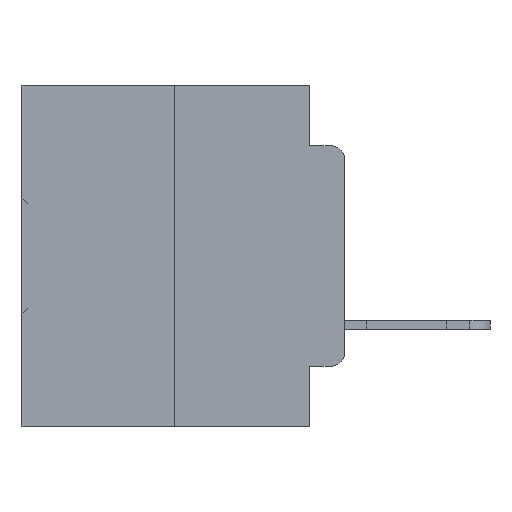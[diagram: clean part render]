
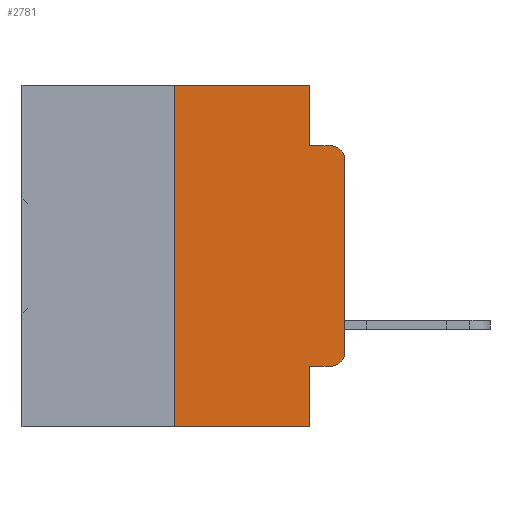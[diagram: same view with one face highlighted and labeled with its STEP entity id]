
A CAD part, left-side view. The second image highlights one B-rep face of the part: STEP entity #2781.
In plain terms, the highlighted planar face has unit normal (-1, 0, 0).
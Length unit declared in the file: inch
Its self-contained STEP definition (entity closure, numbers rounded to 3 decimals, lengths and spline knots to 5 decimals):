
#951 = EDGE_LOOP ( 'NONE', ( #16702, #34845, #14165, #1752, #12583, #24520, #26987, #28486, #2796, #16940 ) ) ;
#1752 = ORIENTED_EDGE ( 'NONE', *, *, #7060, .F. ) ;
#1997 = DIRECTION ( 'NONE',  ( -1., 0., 0. ) ) ;
#2239 = LINE ( 'NONE', #32340, #24091 ) ;
#2675 = DIRECTION ( 'NONE',  ( 0., 0., 1. ) ) ;
#2781 = ADVANCED_FACE ( 'NONE', ( #27780 ), #6393, .F. ) ;
#2796 = ORIENTED_EDGE ( 'NONE', *, *, #31433, .T. ) ;
#2851 = CARTESIAN_POINT ( 'NONE',  ( 0., 0., 0. ) ) ;
#3292 = VERTEX_POINT ( 'NONE', #24514 ) ;
#4327 = LINE ( 'NONE', #14960, #11326 ) ;
#4778 = LINE ( 'NONE', #31733, #27092 ) ;
#4791 = CARTESIAN_POINT ( 'NONE',  ( 0., 0.25, -0.5 ) ) ;
#5276 = VERTEX_POINT ( 'NONE', #4791 ) ;
#6227 = DIRECTION ( 'NONE',  ( 0., 0., -1. ) ) ;
#6255 = VECTOR ( 'NONE', #18401, 39.37008 ) ;
#6272 = DIRECTION ( 'NONE',  ( 1., 0., 0. ) ) ;
#6393 = PLANE ( 'NONE',  #18768 ) ;
#6863 = CARTESIAN_POINT ( 'NONE',  ( 0., 0., -0.3915 ) ) ;
#7060 = EDGE_CURVE ( 'NONE', #3292, #7472, #4778, .T. ) ;
#7232 = CARTESIAN_POINT ( 'NONE',  ( 0., 0.473, 0. ) ) ;
#7472 = VERTEX_POINT ( 'NONE', #17332 ) ;
#7509 = VERTEX_POINT ( 'NONE', #14295 ) ;
#8994 = LINE ( 'NONE', #24898, #15753 ) ;
#8995 = CARTESIAN_POINT ( 'NONE',  ( 0., 0.02, -0.4115 ) ) ;
#10977 = EDGE_CURVE ( 'NONE', #7472, #30550, #12567, .T. ) ;
#11326 = VECTOR ( 'NONE', #28295, 39.37008 ) ;
#12567 = LINE ( 'NONE', #21452, #18228 ) ;
#12583 = ORIENTED_EDGE ( 'NONE', *, *, #30426, .F. ) ;
#12823 = VERTEX_POINT ( 'NONE', #28527 ) ;
#12955 = EDGE_CURVE ( 'NONE', #27573, #30550, #14167, .T. ) ;
#13745 = CARTESIAN_POINT ( 'NONE',  ( 0., 0., -0.1085 ) ) ;
#13796 = VERTEX_POINT ( 'NONE', #8995 ) ;
#14165 = ORIENTED_EDGE ( 'NONE', *, *, #10977, .F. ) ;
#14167 = CIRCLE ( 'NONE', #18147, 0.02 ) ;
#14295 = CARTESIAN_POINT ( 'NONE',  ( 0., 0.051, -0.4115 ) ) ;
#14604 = EDGE_CURVE ( 'NONE', #5276, #29363, #8994, .T. ) ;
#14680 = VECTOR ( 'NONE', #32801, 39.37008 ) ;
#14824 = EDGE_CURVE ( 'NONE', #32777, #27573, #23410, .T. ) ;
#14960 = CARTESIAN_POINT ( 'NONE',  ( 0., 0.473, 0. ) ) ;
#15619 = CARTESIAN_POINT ( 'NONE',  ( 0., 0.051, -0.4115 ) ) ;
#15753 = VECTOR ( 'NONE', #24825, 39.37008 ) ;
#16702 = ORIENTED_EDGE ( 'NONE', *, *, #14824, .T. ) ;
#16940 = ORIENTED_EDGE ( 'NONE', *, *, #22790, .T. ) ;
#17071 = VECTOR ( 'NONE', #2675, 39.37008 ) ;
#17332 = CARTESIAN_POINT ( 'NONE',  ( 0., 0.051, -0.0885 ) ) ;
#18147 = AXIS2_PLACEMENT_3D ( 'NONE', #25422, #25384, #25356 ) ;
#18228 = VECTOR ( 'NONE', #21155, 39.37008 ) ;
#18401 = DIRECTION ( 'NONE',  ( 0., -1., 0. ) ) ;
#18768 = AXIS2_PLACEMENT_3D ( 'NONE', #7232, #6272, #6227 ) ;
#19356 = CARTESIAN_POINT ( 'NONE',  ( 0., 0.02, -0.3915 ) ) ;
#19357 = DIRECTION ( 'NONE',  ( 0., 0., -1. ) ) ;
#20350 = LINE ( 'NONE', #15619, #6255 ) ;
#20753 = CARTESIAN_POINT ( 'NONE',  ( 0., 0.02, -0.0885 ) ) ;
#21155 = DIRECTION ( 'NONE',  ( 0., -1., 0. ) ) ;
#21452 = CARTESIAN_POINT ( 'NONE',  ( 0., 0.051, -0.0885 ) ) ;
#22070 = DIRECTION ( 'NONE',  ( 0., 0., -1. ) ) ;
#22790 = EDGE_CURVE ( 'NONE', #13796, #32777, #27813, .T. ) ;
#23410 = LINE ( 'NONE', #2851, #17071 ) ;
#24091 = VECTOR ( 'NONE', #19357, 39.37008 ) ;
#24514 = CARTESIAN_POINT ( 'NONE',  ( 0., 0.051, 0. ) ) ;
#24520 = ORIENTED_EDGE ( 'NONE', *, *, #34691, .F. ) ;
#24825 = DIRECTION ( 'NONE',  ( 0., -1., 0. ) ) ;
#24898 = CARTESIAN_POINT ( 'NONE',  ( 0., 0.473, -0.5 ) ) ;
#25356 = DIRECTION ( 'NONE',  ( 0., 0., -1. ) ) ;
#25384 = DIRECTION ( 'NONE',  ( -1., 0., 0. ) ) ;
#25422 = CARTESIAN_POINT ( 'NONE',  ( 0., 0.02, -0.1085 ) ) ;
#26987 = ORIENTED_EDGE ( 'NONE', *, *, #14604, .T. ) ;
#27092 = VECTOR ( 'NONE', #31446, 39.37008 ) ;
#27573 = VERTEX_POINT ( 'NONE', #13745 ) ;
#27780 = FACE_OUTER_BOUND ( 'NONE', #951, .T. ) ;
#27813 = CIRCLE ( 'NONE', #31502, 0.02 ) ;
#28295 = DIRECTION ( 'NONE',  ( 0., -1., 0. ) ) ;
#28486 = ORIENTED_EDGE ( 'NONE', *, *, #33092, .F. ) ;
#28527 = CARTESIAN_POINT ( 'NONE',  ( 0., 0.25, 0. ) ) ;
#29363 = VERTEX_POINT ( 'NONE', #29699 ) ;
#29699 = CARTESIAN_POINT ( 'NONE',  ( 0., 0.051, -0.5 ) ) ;
#30426 = EDGE_CURVE ( 'NONE', #12823, #3292, #4327, .T. ) ;
#30481 = LINE ( 'NONE', #35126, #14680 ) ;
#30550 = VERTEX_POINT ( 'NONE', #20753 ) ;
#31433 = EDGE_CURVE ( 'NONE', #7509, #13796, #20350, .T. ) ;
#31446 = DIRECTION ( 'NONE',  ( 0., 0., -1. ) ) ;
#31502 = AXIS2_PLACEMENT_3D ( 'NONE', #19356, #1997, #22070 ) ;
#31733 = CARTESIAN_POINT ( 'NONE',  ( 0., 0.051, 0. ) ) ;
#32340 = CARTESIAN_POINT ( 'NONE',  ( 0., 0.051, 0. ) ) ;
#32777 = VERTEX_POINT ( 'NONE', #6863 ) ;
#32801 = DIRECTION ( 'NONE',  ( 0., 0., 1. ) ) ;
#33092 = EDGE_CURVE ( 'NONE', #7509, #29363, #2239, .T. ) ;
#34691 = EDGE_CURVE ( 'NONE', #5276, #12823, #30481, .T. ) ;
#34845 = ORIENTED_EDGE ( 'NONE', *, *, #12955, .T. ) ;
#35126 = CARTESIAN_POINT ( 'NONE',  ( 0., 0.25, 0. ) ) ;
